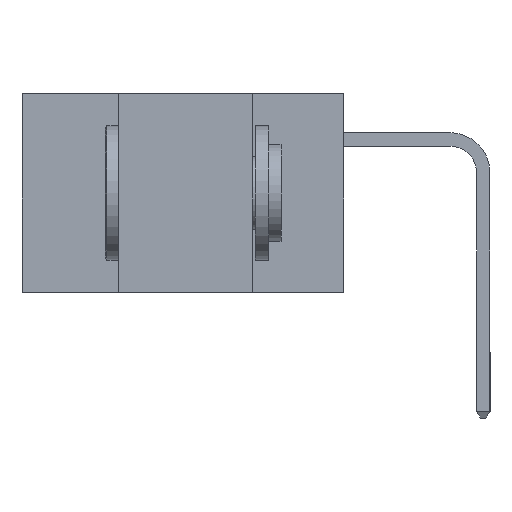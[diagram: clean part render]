
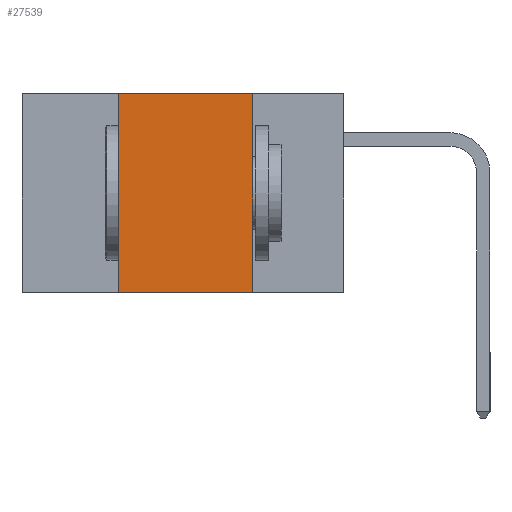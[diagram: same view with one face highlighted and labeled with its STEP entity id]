
A CAD part, left-side view. The second image highlights one B-rep face of the part: STEP entity #27539.
In plain terms, the highlighted planar face has unit normal (-1, 0, 0).
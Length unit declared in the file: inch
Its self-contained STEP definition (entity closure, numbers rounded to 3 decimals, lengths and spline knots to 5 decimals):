
#122 = VERTEX_POINT ( 'NONE', #9482 ) ;
#286 = CARTESIAN_POINT ( 'NONE',  ( 0., 0.17, 0. ) ) ;
#1895 = CARTESIAN_POINT ( 'NONE',  ( 0., 0.6, 0. ) ) ;
#2319 = CARTESIAN_POINT ( 'NONE',  ( 0., 0.17, 0. ) ) ;
#3069 = DIRECTION ( 'NONE',  ( 0., 0., 1. ) ) ;
#3070 = CARTESIAN_POINT ( 'NONE',  ( 0., 0.6, -0.37 ) ) ;
#3221 = VECTOR ( 'NONE', #12919, 39.37008 ) ;
#3446 = CARTESIAN_POINT ( 'NONE',  ( 0., 0.6, 0. ) ) ;
#3483 = LINE ( 'NONE', #5252, #17281 ) ;
#3769 = DIRECTION ( 'NONE',  ( 0., -1., 0. ) ) ;
#5252 = CARTESIAN_POINT ( 'NONE',  ( 0., 0.42, 0. ) ) ;
#5954 = CARTESIAN_POINT ( 'NONE',  ( 0., 0.42, -0.37 ) ) ;
#6850 = LINE ( 'NONE', #286, #11219 ) ;
#7758 = DIRECTION ( 'NONE',  ( 0., 0., -1. ) ) ;
#8549 = VECTOR ( 'NONE', #3769, 39.37008 ) ;
#9482 = CARTESIAN_POINT ( 'NONE',  ( 0., 0.42, 0. ) ) ;
#10349 = ORIENTED_EDGE ( 'NONE', *, *, #18320, .F. ) ;
#11219 = VECTOR ( 'NONE', #13064, 39.37008 ) ;
#11590 = LINE ( 'NONE', #3070, #3221 ) ;
#12638 = EDGE_CURVE ( 'NONE', #21789, #24893, #11590, .T. ) ;
#12919 = DIRECTION ( 'NONE',  ( 0., -1., 0. ) ) ;
#13064 = DIRECTION ( 'NONE',  ( 0., 0., -1. ) ) ;
#13363 = AXIS2_PLACEMENT_3D ( 'NONE', #3446, #20604, #7758 ) ;
#14259 = LINE ( 'NONE', #1895, #8549 ) ;
#16312 = PLANE ( 'NONE',  #13363 ) ;
#17281 = VECTOR ( 'NONE', #3069, 39.37008 ) ;
#18086 = EDGE_CURVE ( 'NONE', #122, #26929, #14259, .T. ) ;
#18222 = ORIENTED_EDGE ( 'NONE', *, *, #18086, .F. ) ;
#18320 = EDGE_CURVE ( 'NONE', #21789, #122, #3483, .T. ) ;
#20021 = FACE_OUTER_BOUND ( 'NONE', #21797, .T. ) ;
#20604 = DIRECTION ( 'NONE',  ( 1., 0., 0. ) ) ;
#21789 = VERTEX_POINT ( 'NONE', #5954 ) ;
#21797 = EDGE_LOOP ( 'NONE', ( #26256, #18222, #10349, #24667 ) ) ;
#22619 = CARTESIAN_POINT ( 'NONE',  ( 0., 0.17, -0.37 ) ) ;
#23688 = EDGE_CURVE ( 'NONE', #26929, #24893, #6850, .T. ) ;
#24667 = ORIENTED_EDGE ( 'NONE', *, *, #12638, .T. ) ;
#24893 = VERTEX_POINT ( 'NONE', #22619 ) ;
#26256 = ORIENTED_EDGE ( 'NONE', *, *, #23688, .F. ) ;
#26929 = VERTEX_POINT ( 'NONE', #2319 ) ;
#27539 = ADVANCED_FACE ( 'NONE', ( #20021 ), #16312, .F. ) ;
